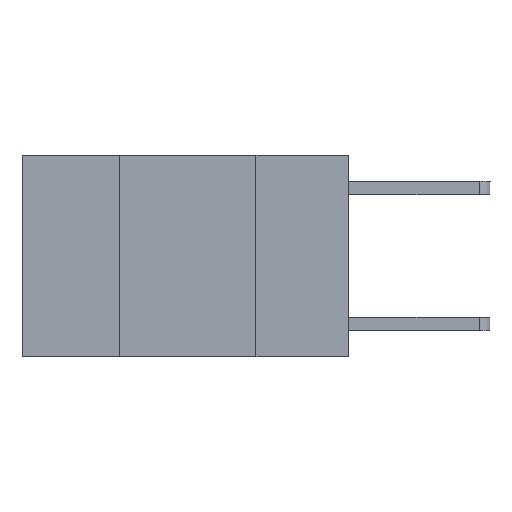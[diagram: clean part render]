
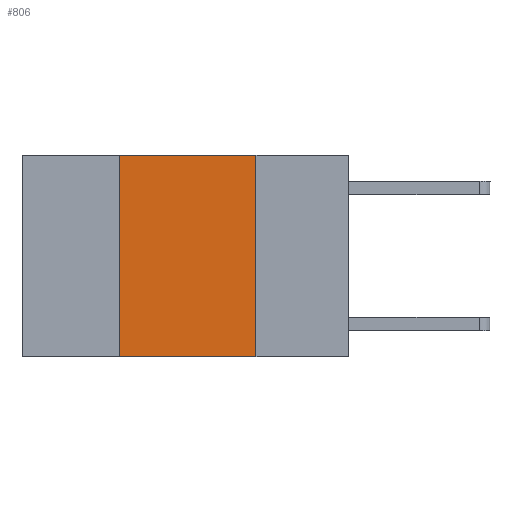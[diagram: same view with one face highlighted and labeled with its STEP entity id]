
A CAD part, left-side view. The second image highlights one B-rep face of the part: STEP entity #806.
In plain terms, the highlighted planar face has unit normal (-1, 0, 0).
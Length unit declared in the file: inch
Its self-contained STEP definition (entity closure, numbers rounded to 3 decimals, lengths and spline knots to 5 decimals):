
#211 = CARTESIAN_POINT ( 'NONE',  ( 0., 0.42, -0.37 ) ) ;
#256 = VECTOR ( 'NONE', #5193, 39.37008 ) ;
#303 = ORIENTED_EDGE ( 'NONE', *, *, #8116, .F. ) ;
#708 = CARTESIAN_POINT ( 'NONE',  ( 0., 0.42, 0. ) ) ;
#806 = ADVANCED_FACE ( 'NONE', ( #5328 ), #4219, .F. ) ;
#864 = VECTOR ( 'NONE', #3319, 39.37008 ) ;
#1083 = CARTESIAN_POINT ( 'NONE',  ( 0., 0.17, 0. ) ) ;
#1201 = VECTOR ( 'NONE', #7437, 39.37008 ) ;
#1268 = LINE ( 'NONE', #2007, #256 ) ;
#1278 = LINE ( 'NONE', #5244, #864 ) ;
#1669 = ORIENTED_EDGE ( 'NONE', *, *, #4559, .T. ) ;
#1701 = VERTEX_POINT ( 'NONE', #708 ) ;
#1718 = ORIENTED_EDGE ( 'NONE', *, *, #7049, .F. ) ;
#1728 = DIRECTION ( 'NONE',  ( 0., 0., 1. ) ) ;
#2007 = CARTESIAN_POINT ( 'NONE',  ( 0., 0.17, 0. ) ) ;
#2012 = VECTOR ( 'NONE', #1728, 39.37008 ) ;
#2089 = EDGE_CURVE ( 'NONE', #3236, #6548, #1268, .T. ) ;
#2335 = CARTESIAN_POINT ( 'NONE',  ( 0., 0.42, 0. ) ) ;
#3236 = VERTEX_POINT ( 'NONE', #1083 ) ;
#3319 = DIRECTION ( 'NONE',  ( 0., -1., 0. ) ) ;
#4015 = DIRECTION ( 'NONE',  ( 0., 0., -1. ) ) ;
#4191 = LINE ( 'NONE', #8245, #1201 ) ;
#4219 = PLANE ( 'NONE',  #4398 ) ;
#4398 = AXIS2_PLACEMENT_3D ( 'NONE', #7898, #7224, #4015 ) ;
#4559 = EDGE_CURVE ( 'NONE', #6510, #6548, #1278, .T. ) ;
#5193 = DIRECTION ( 'NONE',  ( 0., 0., -1. ) ) ;
#5244 = CARTESIAN_POINT ( 'NONE',  ( 0., 0.6, -0.37 ) ) ;
#5328 = FACE_OUTER_BOUND ( 'NONE', #6915, .T. ) ;
#5462 = ORIENTED_EDGE ( 'NONE', *, *, #2089, .F. ) ;
#6279 = CARTESIAN_POINT ( 'NONE',  ( 0., 0.17, -0.37 ) ) ;
#6510 = VERTEX_POINT ( 'NONE', #211 ) ;
#6548 = VERTEX_POINT ( 'NONE', #6279 ) ;
#6915 = EDGE_LOOP ( 'NONE', ( #5462, #303, #1718, #1669 ) ) ;
#7049 = EDGE_CURVE ( 'NONE', #6510, #1701, #7615, .T. ) ;
#7224 = DIRECTION ( 'NONE',  ( 1., 0., 0. ) ) ;
#7437 = DIRECTION ( 'NONE',  ( 0., -1., 0. ) ) ;
#7615 = LINE ( 'NONE', #2335, #2012 ) ;
#7898 = CARTESIAN_POINT ( 'NONE',  ( 0., 0.6, 0. ) ) ;
#8116 = EDGE_CURVE ( 'NONE', #1701, #3236, #4191, .T. ) ;
#8245 = CARTESIAN_POINT ( 'NONE',  ( 0., 0.6, 0. ) ) ;
